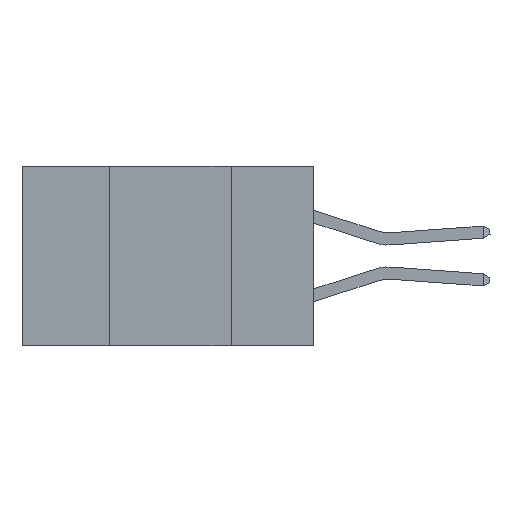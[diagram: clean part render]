
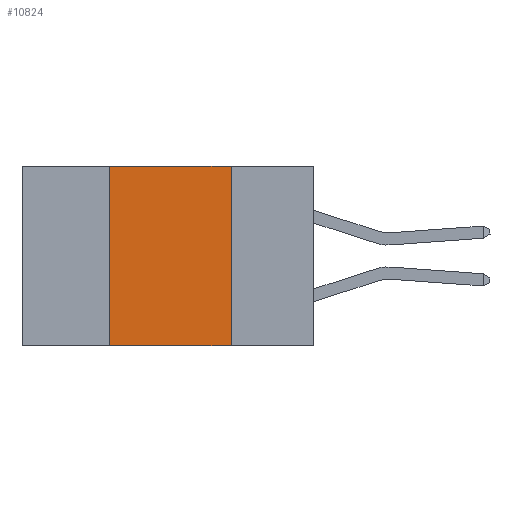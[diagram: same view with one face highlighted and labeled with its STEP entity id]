
A CAD part, left-side view. The second image highlights one B-rep face of the part: STEP entity #10824.
In plain terms, the highlighted planar face has unit normal (-1, 0, 0).
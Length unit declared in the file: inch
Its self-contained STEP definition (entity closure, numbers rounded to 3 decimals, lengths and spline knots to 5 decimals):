
#770 = ORIENTED_EDGE ( 'NONE', *, *, #11670, .F. ) ;
#2809 = VERTEX_POINT ( 'NONE', #21935 ) ;
#2961 = DIRECTION ( 'NONE',  ( 0., -1., 0. ) ) ;
#3400 = CARTESIAN_POINT ( 'NONE',  ( 0., 0.17, 0. ) ) ;
#3564 = LINE ( 'NONE', #26436, #7597 ) ;
#4176 = DIRECTION ( 'NONE',  ( 0., -1., 0. ) ) ;
#4721 = LINE ( 'NONE', #16165, #9829 ) ;
#4833 = EDGE_LOOP ( 'NONE', ( #13890, #770, #26041, #10387 ) ) ;
#6093 = LINE ( 'NONE', #24283, #29039 ) ;
#6948 = AXIS2_PLACEMENT_3D ( 'NONE', #12905, #22166, #10565 ) ;
#7597 = VECTOR ( 'NONE', #2961, 39.37008 ) ;
#9477 = CARTESIAN_POINT ( 'NONE',  ( 0., 0.42, -0.37 ) ) ;
#9829 = VECTOR ( 'NONE', #15875, 39.37008 ) ;
#10240 = CARTESIAN_POINT ( 'NONE',  ( 0., 0.17, 0. ) ) ;
#10387 = ORIENTED_EDGE ( 'NONE', *, *, #17358, .T. ) ;
#10565 = DIRECTION ( 'NONE',  ( 0., 0., -1. ) ) ;
#10824 = ADVANCED_FACE ( 'NONE', ( #26428 ), #13196, .F. ) ;
#11356 = VECTOR ( 'NONE', #25668, 39.37008 ) ;
#11670 = EDGE_CURVE ( 'NONE', #23154, #21947, #6093, .T. ) ;
#12905 = CARTESIAN_POINT ( 'NONE',  ( 0., 0.6, 0. ) ) ;
#13196 = PLANE ( 'NONE',  #6948 ) ;
#13890 = ORIENTED_EDGE ( 'NONE', *, *, #17750, .F. ) ;
#14883 = EDGE_CURVE ( 'NONE', #22512, #23154, #4721, .T. ) ;
#15875 = DIRECTION ( 'NONE',  ( 0., 0., 1. ) ) ;
#16165 = CARTESIAN_POINT ( 'NONE',  ( 0., 0.42, 0. ) ) ;
#16702 = LINE ( 'NONE', #10240, #11356 ) ;
#17358 = EDGE_CURVE ( 'NONE', #22512, #2809, #3564, .T. ) ;
#17750 = EDGE_CURVE ( 'NONE', #21947, #2809, #16702, .T. ) ;
#21935 = CARTESIAN_POINT ( 'NONE',  ( 0., 0.17, -0.37 ) ) ;
#21947 = VERTEX_POINT ( 'NONE', #3400 ) ;
#22166 = DIRECTION ( 'NONE',  ( 1., 0., 0. ) ) ;
#22512 = VERTEX_POINT ( 'NONE', #9477 ) ;
#23154 = VERTEX_POINT ( 'NONE', #25599 ) ;
#24283 = CARTESIAN_POINT ( 'NONE',  ( 0., 0.6, 0. ) ) ;
#25599 = CARTESIAN_POINT ( 'NONE',  ( 0., 0.42, 0. ) ) ;
#25668 = DIRECTION ( 'NONE',  ( 0., 0., -1. ) ) ;
#26041 = ORIENTED_EDGE ( 'NONE', *, *, #14883, .F. ) ;
#26428 = FACE_OUTER_BOUND ( 'NONE', #4833, .T. ) ;
#26436 = CARTESIAN_POINT ( 'NONE',  ( 0., 0.6, -0.37 ) ) ;
#29039 = VECTOR ( 'NONE', #4176, 39.37008 ) ;
